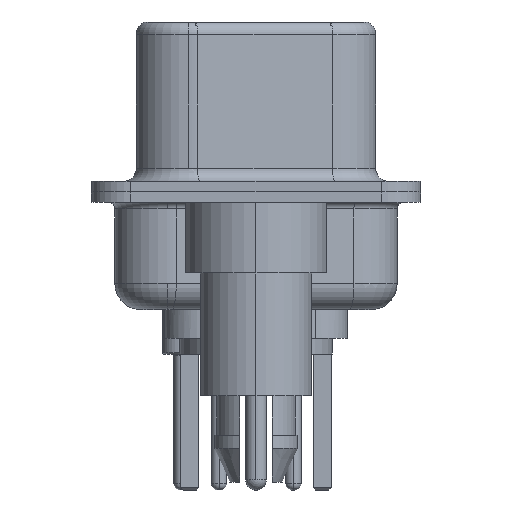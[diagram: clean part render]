
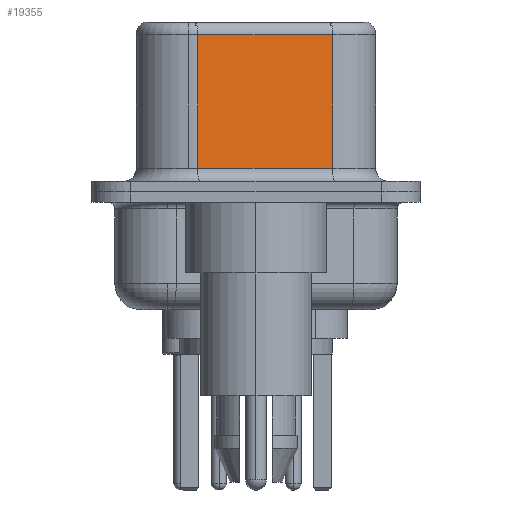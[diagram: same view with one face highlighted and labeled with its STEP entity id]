
A CAD part, left-side view. The second image highlights one B-rep face of the part: STEP entity #19355.
In plain terms, the highlighted planar face has unit normal (-0.985, -0.174, 0).
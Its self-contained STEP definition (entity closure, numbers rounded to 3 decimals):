
#165 = VECTOR ( 'NONE', #14429, 1000. ) ;
#582 = ORIENTED_EDGE ( 'NONE', *, *, #25990, .F. ) ;
#1124 = EDGE_CURVE ( 'NONE', #9230, #13533, #14002, .T. ) ;
#2208 = ORIENTED_EDGE ( 'NONE', *, *, #1124, .T. ) ;
#2710 = LINE ( 'NONE', #7977, #18518 ) ;
#3361 = CARTESIAN_POINT ( 'NONE',  ( 3.67, 2.233, 6.02 ) ) ;
#4476 = VECTOR ( 'NONE', #22856, 1000. ) ;
#4953 = ORIENTED_EDGE ( 'NONE', *, *, #11880, .T. ) ;
#5406 = VERTEX_POINT ( 'NONE', #3361 ) ;
#5834 = DIRECTION ( 'NONE',  ( -0.174, 0.985, 0. ) ) ;
#6781 = DIRECTION ( 'NONE',  ( -0.174, 0.985, 0. ) ) ;
#7977 = CARTESIAN_POINT ( 'NONE',  ( 4.58, -2.927, 6.02 ) ) ;
#8989 = VECTOR ( 'NONE', #20670, 1000. ) ;
#9230 = VERTEX_POINT ( 'NONE', #23118 ) ;
#9475 = LINE ( 'NONE', #25092, #4476 ) ;
#10019 = CARTESIAN_POINT ( 'NONE',  ( 4.58, -2.927, 6.02 ) ) ;
#10398 = EDGE_CURVE ( 'NONE', #5406, #9230, #9475, .T. ) ;
#10870 = EDGE_LOOP ( 'NONE', ( #582, #4953, #20993, #2208 ) ) ;
#11880 = EDGE_CURVE ( 'NONE', #24245, #5406, #2710, .T. ) ;
#13431 = CARTESIAN_POINT ( 'NONE',  ( 4.58, -2.927, 0.9 ) ) ;
#13533 = VERTEX_POINT ( 'NONE', #16398 ) ;
#14002 = LINE ( 'NONE', #13431, #8989 ) ;
#14429 = DIRECTION ( 'NONE',  ( 0., 0., -1. ) ) ;
#15478 = FACE_OUTER_BOUND ( 'NONE', #10870, .T. ) ;
#16398 = CARTESIAN_POINT ( 'NONE',  ( 4.58, -2.927, 0.9 ) ) ;
#18518 = VECTOR ( 'NONE', #5834, 1000. ) ;
#19355 = ADVANCED_FACE ( 'NONE', ( #15478 ), #21661, .F. ) ;
#19634 = DIRECTION ( 'NONE',  ( 0.985, 0.174, 0. ) ) ;
#20670 = DIRECTION ( 'NONE',  ( 0.174, -0.985, 0. ) ) ;
#20749 = CARTESIAN_POINT ( 'NONE',  ( 4.58, -2.927, 6.52 ) ) ;
#20993 = ORIENTED_EDGE ( 'NONE', *, *, #10398, .T. ) ;
#21661 = PLANE ( 'NONE',  #26395 ) ;
#22769 = LINE ( 'NONE', #20749, #165 ) ;
#22856 = DIRECTION ( 'NONE',  ( 0., 0., -1. ) ) ;
#23118 = CARTESIAN_POINT ( 'NONE',  ( 3.67, 2.233, 0.9 ) ) ;
#24245 = VERTEX_POINT ( 'NONE', #10019 ) ;
#25092 = CARTESIAN_POINT ( 'NONE',  ( 3.67, 2.233, 6.52 ) ) ;
#25990 = EDGE_CURVE ( 'NONE', #24245, #13533, #22769, .T. ) ;
#25999 = CARTESIAN_POINT ( 'NONE',  ( 4.58, -2.927, 6.52 ) ) ;
#26395 = AXIS2_PLACEMENT_3D ( 'NONE', #25999, #19634, #6781 ) ;
